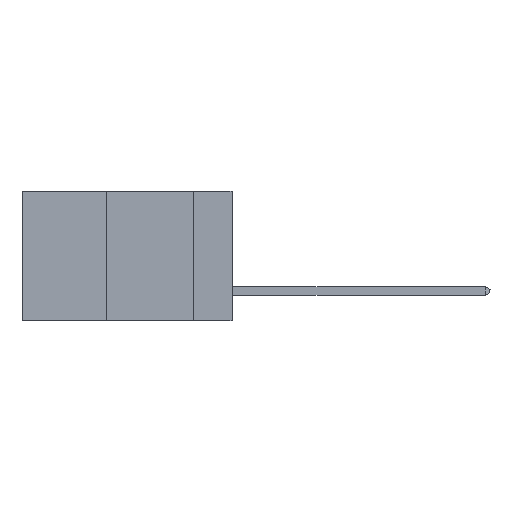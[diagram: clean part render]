
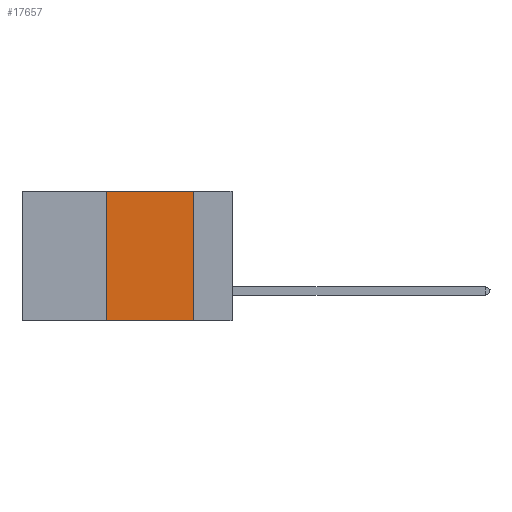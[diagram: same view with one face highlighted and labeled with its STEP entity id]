
A CAD part, left-side view. The second image highlights one B-rep face of the part: STEP entity #17657.
In plain terms, the highlighted planar face has unit normal (-1, 0, 0).
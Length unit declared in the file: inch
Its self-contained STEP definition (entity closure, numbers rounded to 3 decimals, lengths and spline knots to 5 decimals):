
#1087 = EDGE_CURVE ( 'NONE', #18687, #11479, #28160, .T. ) ;
#1694 = CARTESIAN_POINT ( 'NONE',  ( 0., 0.11, 0. ) ) ;
#2126 = EDGE_LOOP ( 'NONE', ( #8834, #22335, #18732, #13433 ) ) ;
#3998 = FACE_OUTER_BOUND ( 'NONE', #2126, .T. ) ;
#4556 = LINE ( 'NONE', #22978, #18884 ) ;
#4693 = DIRECTION ( 'NONE',  ( 0., 0., 1. ) ) ;
#5663 = CARTESIAN_POINT ( 'NONE',  ( 0., 0.36, 0. ) ) ;
#6966 = EDGE_CURVE ( 'NONE', #11479, #25025, #9506, .T. ) ;
#6994 = EDGE_CURVE ( 'NONE', #18687, #21825, #4556, .T. ) ;
#7428 = VECTOR ( 'NONE', #4693, 39.37008 ) ;
#7845 = CARTESIAN_POINT ( 'NONE',  ( 0., 0.6, 0. ) ) ;
#8834 = ORIENTED_EDGE ( 'NONE', *, *, #29758, .F. ) ;
#9069 = CARTESIAN_POINT ( 'NONE',  ( 0., 0.11, -0.37 ) ) ;
#9506 = LINE ( 'NONE', #15383, #16331 ) ;
#11479 = VERTEX_POINT ( 'NONE', #5663 ) ;
#11776 = VECTOR ( 'NONE', #30098, 39.37008 ) ;
#12039 = CARTESIAN_POINT ( 'NONE',  ( 0., 0.36, 0. ) ) ;
#13433 = ORIENTED_EDGE ( 'NONE', *, *, #6994, .T. ) ;
#14851 = DIRECTION ( 'NONE',  ( 0., 0., -1. ) ) ;
#15383 = CARTESIAN_POINT ( 'NONE',  ( 0., 0.6, 0. ) ) ;
#15544 = LINE ( 'NONE', #24918, #11776 ) ;
#16331 = VECTOR ( 'NONE', #17766, 39.37008 ) ;
#17657 = ADVANCED_FACE ( 'NONE', ( #3998 ), #29495, .F. ) ;
#17766 = DIRECTION ( 'NONE',  ( 0., -1., 0. ) ) ;
#18687 = VERTEX_POINT ( 'NONE', #19683 ) ;
#18732 = ORIENTED_EDGE ( 'NONE', *, *, #1087, .F. ) ;
#18884 = VECTOR ( 'NONE', #25193, 39.37008 ) ;
#19683 = CARTESIAN_POINT ( 'NONE',  ( 0., 0.36, -0.37 ) ) ;
#21825 = VERTEX_POINT ( 'NONE', #9069 ) ;
#22335 = ORIENTED_EDGE ( 'NONE', *, *, #6966, .F. ) ;
#22978 = CARTESIAN_POINT ( 'NONE',  ( 0., 0.6, -0.37 ) ) ;
#23352 = AXIS2_PLACEMENT_3D ( 'NONE', #7845, #27195, #14851 ) ;
#24918 = CARTESIAN_POINT ( 'NONE',  ( 0., 0.11, 0. ) ) ;
#25025 = VERTEX_POINT ( 'NONE', #1694 ) ;
#25193 = DIRECTION ( 'NONE',  ( 0., -1., 0. ) ) ;
#27195 = DIRECTION ( 'NONE',  ( 1., 0., 0. ) ) ;
#28160 = LINE ( 'NONE', #12039, #7428 ) ;
#29495 = PLANE ( 'NONE',  #23352 ) ;
#29758 = EDGE_CURVE ( 'NONE', #25025, #21825, #15544, .T. ) ;
#30098 = DIRECTION ( 'NONE',  ( 0., 0., -1. ) ) ;
